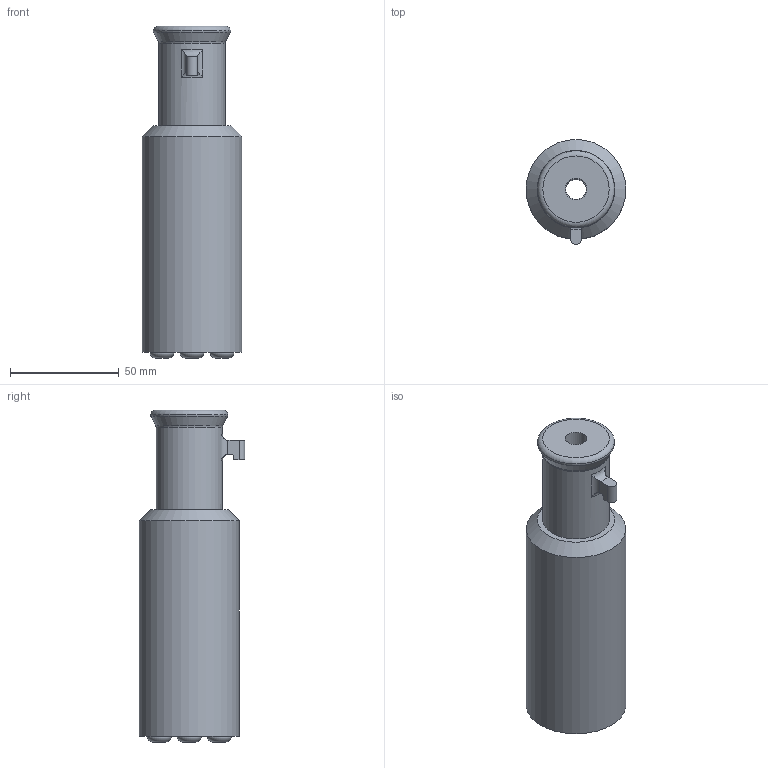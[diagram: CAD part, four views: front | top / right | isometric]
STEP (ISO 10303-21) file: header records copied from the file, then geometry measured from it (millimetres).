
FILE_DESCRIPTION((' '),'2;1');
FILE_NAME('Hydrabarrel1.stp','2013-06-04T21:39:34',(' '),(' '),' ','ACIS',' ');
FILE_SCHEMA(('CONFIG_CONTROL_DESIGN'));
Length unit declared in the file: inch
Products named in the file (1): Hydrabarrel1.stp
Bounding box: 45.77 x 48.29 x 152.4 mm (x, y, z)
Volume: 194840.6 mm3; surface area: 27228 mm2
Topology: 1 solids, 1 shells, 51 faces, 123 edges, 80 vertices
Faces by surface type: plane 28, torus 12, cylinder 9, cone 2
Full cylindrical faces by diameter (mm): 9.398 x1, 9.906 x1, 30.48 x1, 45.771 x1
Entity records: 1558 total; most frequent: CARTESIAN_POINT 295, DIRECTION 249, ORIENTED_EDGE 212, EDGE_CURVE 106, AXIS2_PLACEMENT_3D 97, VERTEX_POINT 77, EDGE_LOOP 73, VECTOR 55
